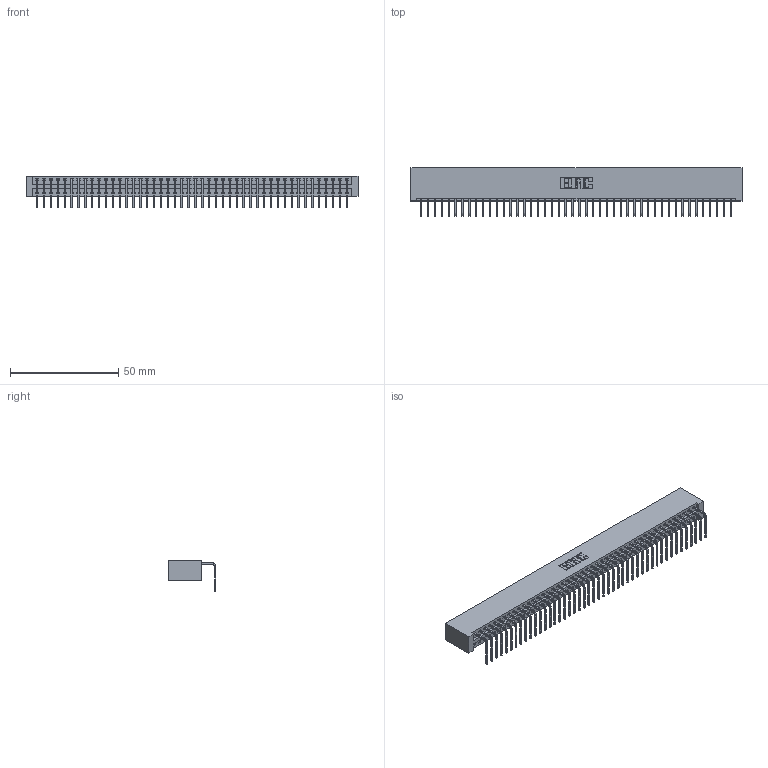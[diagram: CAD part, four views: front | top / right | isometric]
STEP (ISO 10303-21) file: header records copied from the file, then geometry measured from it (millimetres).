
FILE_DESCRIPTION (( 'STEP AP203' ), '1' );
FILE_NAME ('396-046-558-101.STEP', '2019-11-01T08:15:41', ( '' ), ( '' ), 'SwSTEP 2.0', 'SolidWorks 2016', '' );
FILE_SCHEMA (( 'CONFIG_CONTROL_DESIGN' ));
Length unit declared in the file: inch
Products named in the file (3): 346 Part_No Mounting Lugs; 345-292-001_558 Tail - 2; 396-046-558-101
Assembly tree (47 placements, depth 2):
  396-046-558-101
    346 Part_No Mounting Lugs
    345-292-001_558 Tail - 2  x46
Bounding box: 153.29 x 22.16 x 14.73 mm (x, y, z)
Volume: 15403.4 mm3; surface area: 20284.8 mm2
Topology: 47 solids, 47 shells, 2874 faces, 8677 edges, 5722 vertices
Faces by surface type: plane 2004, cylinder 870
Entity records: 27817 total; most frequent: CARTESIAN_POINT 4774, ORIENTED_EDGE 4754, DIRECTION 4201, EDGE_CURVE 2377, VECTOR 2069, LINE 2069, VERTEX_POINT 1582, AXIS2_PLACEMENT_3D 1066
